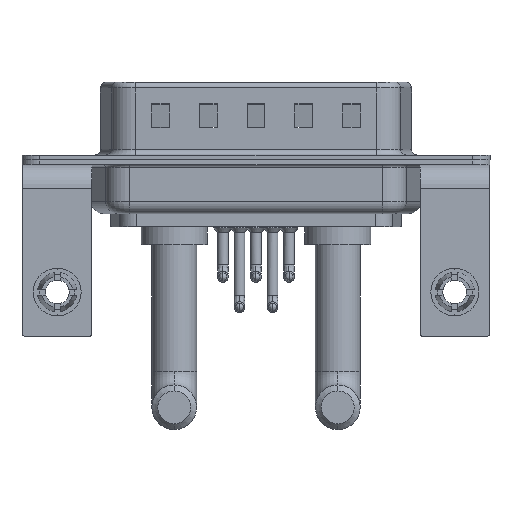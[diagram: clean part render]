
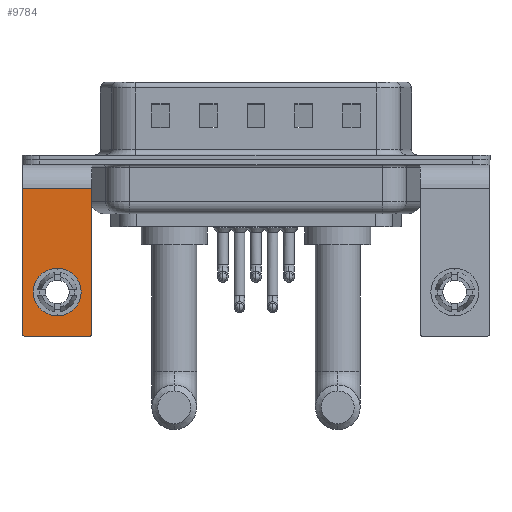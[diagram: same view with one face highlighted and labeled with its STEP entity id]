
A CAD part, front view. The second image highlights one B-rep face of the part: STEP entity #9784.
In plain terms, the highlighted planar face has unit normal (0, -1, 0).
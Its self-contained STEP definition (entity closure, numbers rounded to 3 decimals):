
#39 = CARTESIAN_POINT ( 'NONE',  ( -2.65, -6.25, -14.55 ) ) ;
#51 = LINE ( 'NONE', #10585, #2142 ) ;
#467 = DIRECTION ( 'NONE',  ( -1., 0., 0. ) ) ;
#884 = FACE_BOUND ( 'NONE', #17013, .T. ) ;
#1324 = ORIENTED_EDGE ( 'NONE', *, *, #15995, .T. ) ;
#1609 = DIRECTION ( 'NONE',  ( 0., 1., 0. ) ) ;
#1928 = DIRECTION ( 'NONE',  ( 0., -1., 0. ) ) ;
#2142 = VECTOR ( 'NONE', #10695, 1000. ) ;
#2406 = CARTESIAN_POINT ( 'NONE',  ( -2.9, -6.25, -2.4 ) ) ;
#2947 = CIRCLE ( 'NONE', #15390, 2. ) ;
#3221 = AXIS2_PLACEMENT_3D ( 'NONE', #39, #1928, #14694 ) ;
#3695 = ORIENTED_EDGE ( 'NONE', *, *, #14998, .T. ) ;
#4062 = AXIS2_PLACEMENT_3D ( 'NONE', #14301, #9197, #6955 ) ;
#4098 = PLANE ( 'NONE',  #13677 ) ;
#4110 = VERTEX_POINT ( 'NONE', #12234 ) ;
#4526 = EDGE_LOOP ( 'NONE', ( #20677, #3695, #16555, #4934, #15518, #1324 ) ) ;
#4849 = EDGE_CURVE ( 'NONE', #12853, #20596, #17897, .T. ) ;
#4934 = ORIENTED_EDGE ( 'NONE', *, *, #22502, .T. ) ;
#5044 = EDGE_CURVE ( 'NONE', #11654, #12127, #17186, .T. ) ;
#5166 = CARTESIAN_POINT ( 'NONE',  ( 2.9, -6.25, -14.8 ) ) ;
#5271 = CARTESIAN_POINT ( 'NONE',  ( 2.9, -6.25, -14.55 ) ) ;
#5902 = VECTOR ( 'NONE', #467, 1000. ) ;
#6041 = DIRECTION ( 'NONE',  ( 0., 1., 0. ) ) ;
#6220 = CIRCLE ( 'NONE', #3221, 0.25 ) ;
#6467 = ORIENTED_EDGE ( 'NONE', *, *, #20487, .T. ) ;
#6522 = EDGE_CURVE ( 'NONE', #13804, #16799, #51, .T. ) ;
#6955 = DIRECTION ( 'NONE',  ( 0., 0., 1. ) ) ;
#7792 = CARTESIAN_POINT ( 'NONE',  ( 2.9, -6.25, -2.4 ) ) ;
#9022 = CIRCLE ( 'NONE', #22178, 2. ) ;
#9197 = DIRECTION ( 'NONE',  ( 0., -1., 0. ) ) ;
#9644 = CARTESIAN_POINT ( 'NONE',  ( 2.9, -6.25, -2.4 ) ) ;
#9784 = ADVANCED_FACE ( 'NONE', ( #884, #18827 ), #4098, .F. ) ;
#10367 = DIRECTION ( 'NONE',  ( 0., 0., 1. ) ) ;
#10585 = CARTESIAN_POINT ( 'NONE',  ( 2.9, -6.25, -2.4 ) ) ;
#10695 = DIRECTION ( 'NONE',  ( 0., 0., -1. ) ) ;
#11497 = DIRECTION ( 'NONE',  ( 0., 0., 1. ) ) ;
#11654 = VERTEX_POINT ( 'NONE', #2406 ) ;
#12084 = CARTESIAN_POINT ( 'NONE',  ( -2.9, -6.25, -14.55 ) ) ;
#12127 = VERTEX_POINT ( 'NONE', #12084 ) ;
#12234 = CARTESIAN_POINT ( 'NONE',  ( 0., -6.25, -13.07 ) ) ;
#12853 = VERTEX_POINT ( 'NONE', #22382 ) ;
#12862 = DIRECTION ( 'NONE',  ( -1., 0., 0. ) ) ;
#12969 = DIRECTION ( 'NONE',  ( 0., 1., 0. ) ) ;
#13099 = CIRCLE ( 'NONE', #4062, 0.25 ) ;
#13513 = CARTESIAN_POINT ( 'NONE',  ( -2.65, -6.25, -14.8 ) ) ;
#13644 = VECTOR ( 'NONE', #19188, 1000. ) ;
#13677 = AXIS2_PLACEMENT_3D ( 'NONE', #9644, #12969, #18476 ) ;
#13804 = VERTEX_POINT ( 'NONE', #17241 ) ;
#14301 = CARTESIAN_POINT ( 'NONE',  ( 2.65, -6.25, -14.55 ) ) ;
#14694 = DIRECTION ( 'NONE',  ( 0., 0., 1. ) ) ;
#14998 = EDGE_CURVE ( 'NONE', #12127, #20596, #6220, .T. ) ;
#15390 = AXIS2_PLACEMENT_3D ( 'NONE', #19533, #1609, #10367 ) ;
#15428 = CARTESIAN_POINT ( 'NONE',  ( -2.9, -6.25, -2.4 ) ) ;
#15518 = ORIENTED_EDGE ( 'NONE', *, *, #6522, .F. ) ;
#15995 = EDGE_CURVE ( 'NONE', #13804, #11654, #19605, .T. ) ;
#16063 = CARTESIAN_POINT ( 'NONE',  ( 0., -6.25, -9.07 ) ) ;
#16555 = ORIENTED_EDGE ( 'NONE', *, *, #4849, .F. ) ;
#16799 = VERTEX_POINT ( 'NONE', #5271 ) ;
#16886 = EDGE_CURVE ( 'NONE', #4110, #17873, #2947, .T. ) ;
#17013 = EDGE_LOOP ( 'NONE', ( #17625, #6467 ) ) ;
#17186 = LINE ( 'NONE', #15428, #13644 ) ;
#17241 = CARTESIAN_POINT ( 'NONE',  ( 2.9, -6.25, -2.4 ) ) ;
#17625 = ORIENTED_EDGE ( 'NONE', *, *, #16886, .T. ) ;
#17873 = VERTEX_POINT ( 'NONE', #16063 ) ;
#17897 = LINE ( 'NONE', #5166, #21143 ) ;
#18317 = CARTESIAN_POINT ( 'NONE',  ( 0., -6.25, -11.07 ) ) ;
#18476 = DIRECTION ( 'NONE',  ( 0., 0., 1. ) ) ;
#18827 = FACE_OUTER_BOUND ( 'NONE', #4526, .T. ) ;
#19188 = DIRECTION ( 'NONE',  ( 0., 0., -1. ) ) ;
#19533 = CARTESIAN_POINT ( 'NONE',  ( 0., -6.25, -11.07 ) ) ;
#19605 = LINE ( 'NONE', #7792, #5902 ) ;
#20487 = EDGE_CURVE ( 'NONE', #17873, #4110, #9022, .T. ) ;
#20596 = VERTEX_POINT ( 'NONE', #13513 ) ;
#20677 = ORIENTED_EDGE ( 'NONE', *, *, #5044, .T. ) ;
#21143 = VECTOR ( 'NONE', #12862, 1000. ) ;
#22178 = AXIS2_PLACEMENT_3D ( 'NONE', #18317, #6041, #11497 ) ;
#22382 = CARTESIAN_POINT ( 'NONE',  ( 2.65, -6.25, -14.8 ) ) ;
#22502 = EDGE_CURVE ( 'NONE', #12853, #16799, #13099, .T. ) ;
